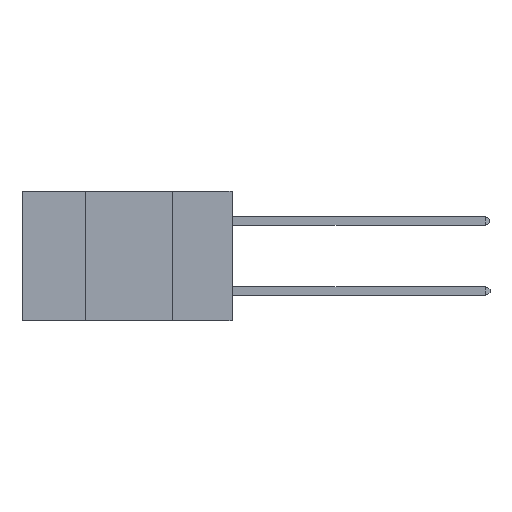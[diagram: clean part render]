
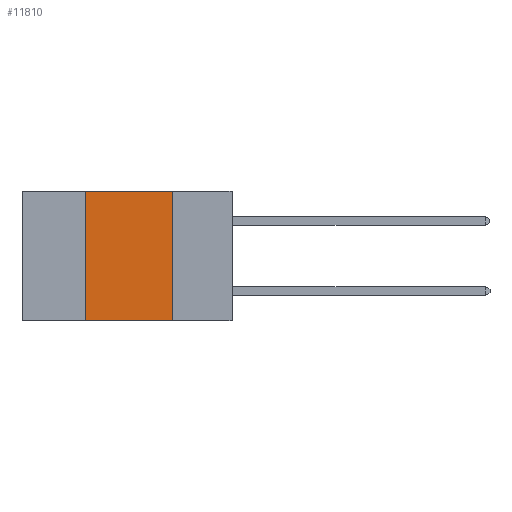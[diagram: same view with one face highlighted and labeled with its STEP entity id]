
A CAD part, left-side view. The second image highlights one B-rep face of the part: STEP entity #11810.
In plain terms, the highlighted planar face has unit normal (-1, 0, 0).
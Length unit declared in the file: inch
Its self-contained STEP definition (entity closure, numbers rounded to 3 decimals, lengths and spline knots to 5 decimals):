
#1676 = LINE ( 'NONE', #12624, #7489 ) ;
#1838 = VERTEX_POINT ( 'NONE', #4374 ) ;
#2229 = CARTESIAN_POINT ( 'NONE',  ( 0., 0.42, 0. ) ) ;
#2283 = DIRECTION ( 'NONE',  ( 0., 0., 1. ) ) ;
#2804 = VECTOR ( 'NONE', #12441, 39.37008 ) ;
#2915 = DIRECTION ( 'NONE',  ( 1., 0., 0. ) ) ;
#3005 = CARTESIAN_POINT ( 'NONE',  ( 0., 0.42, 0. ) ) ;
#3032 = AXIS2_PLACEMENT_3D ( 'NONE', #13447, #2915, #10593 ) ;
#3338 = EDGE_CURVE ( 'NONE', #7903, #12481, #11235, .T. ) ;
#4187 = FACE_OUTER_BOUND ( 'NONE', #7300, .T. ) ;
#4374 = CARTESIAN_POINT ( 'NONE',  ( 0., 0.17, -0.37 ) ) ;
#5675 = VECTOR ( 'NONE', #2283, 39.37008 ) ;
#6379 = VERTEX_POINT ( 'NONE', #10335 ) ;
#7300 = EDGE_LOOP ( 'NONE', ( #8160, #12478, #13364, #11825 ) ) ;
#7409 = VECTOR ( 'NONE', #13310, 39.37008 ) ;
#7489 = VECTOR ( 'NONE', #7651, 39.37008 ) ;
#7638 = EDGE_CURVE ( 'NONE', #12481, #6379, #13709, .T. ) ;
#7651 = DIRECTION ( 'NONE',  ( 0., -1., 0. ) ) ;
#7903 = VERTEX_POINT ( 'NONE', #9923 ) ;
#8160 = ORIENTED_EDGE ( 'NONE', *, *, #13217, .F. ) ;
#8467 = EDGE_CURVE ( 'NONE', #7903, #1838, #1676, .T. ) ;
#9491 = CARTESIAN_POINT ( 'NONE',  ( 0., 0.6, 0. ) ) ;
#9923 = CARTESIAN_POINT ( 'NONE',  ( 0., 0.42, -0.37 ) ) ;
#10335 = CARTESIAN_POINT ( 'NONE',  ( 0., 0.17, 0. ) ) ;
#10554 = PLANE ( 'NONE',  #3032 ) ;
#10593 = DIRECTION ( 'NONE',  ( 0., 0., -1. ) ) ;
#11235 = LINE ( 'NONE', #2229, #5675 ) ;
#11810 = ADVANCED_FACE ( 'NONE', ( #4187 ), #10554, .F. ) ;
#11825 = ORIENTED_EDGE ( 'NONE', *, *, #8467, .T. ) ;
#12369 = CARTESIAN_POINT ( 'NONE',  ( 0., 0.17, 0. ) ) ;
#12441 = DIRECTION ( 'NONE',  ( 0., -1., 0. ) ) ;
#12478 = ORIENTED_EDGE ( 'NONE', *, *, #7638, .F. ) ;
#12481 = VERTEX_POINT ( 'NONE', #3005 ) ;
#12624 = CARTESIAN_POINT ( 'NONE',  ( 0., 0.6, -0.37 ) ) ;
#12745 = LINE ( 'NONE', #12369, #7409 ) ;
#13217 = EDGE_CURVE ( 'NONE', #6379, #1838, #12745, .T. ) ;
#13310 = DIRECTION ( 'NONE',  ( 0., 0., -1. ) ) ;
#13364 = ORIENTED_EDGE ( 'NONE', *, *, #3338, .F. ) ;
#13447 = CARTESIAN_POINT ( 'NONE',  ( 0., 0.6, 0. ) ) ;
#13709 = LINE ( 'NONE', #9491, #2804 ) ;
